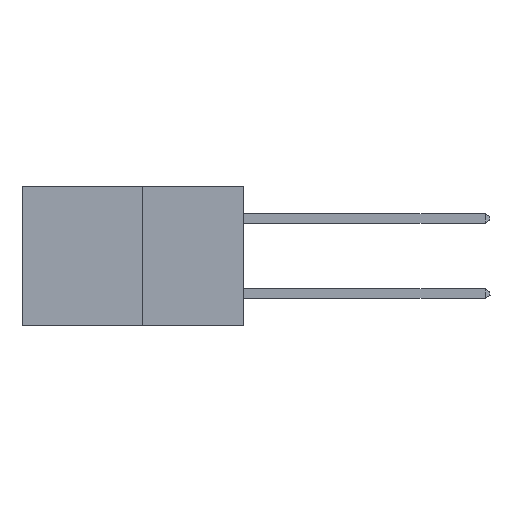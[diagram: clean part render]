
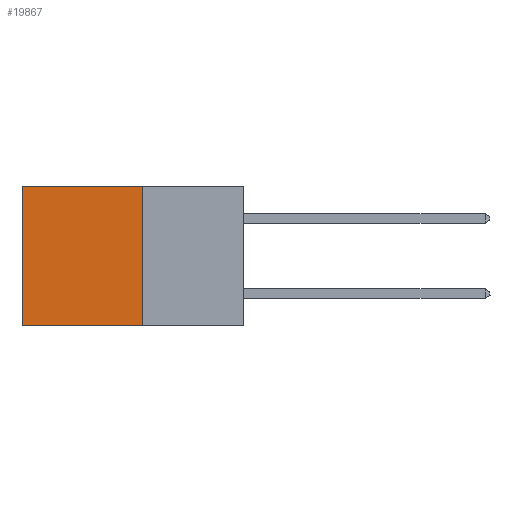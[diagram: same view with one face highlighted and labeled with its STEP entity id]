
A CAD part, left-side view. The second image highlights one B-rep face of the part: STEP entity #19867.
In plain terms, the highlighted planar face has unit normal (-1, 0, 0).
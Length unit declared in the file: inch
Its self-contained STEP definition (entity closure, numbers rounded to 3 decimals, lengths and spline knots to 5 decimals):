
#565 = DIRECTION ( 'NONE',  ( 0., 0., -1. ) ) ;
#991 = LINE ( 'NONE', #5631, #18866 ) ;
#1323 = ORIENTED_EDGE ( 'NONE', *, *, #17153, .F. ) ;
#2403 = CARTESIAN_POINT ( 'NONE',  ( 0.277, 0.27, -0.37 ) ) ;
#3775 = VERTEX_POINT ( 'NONE', #9817 ) ;
#5423 = CARTESIAN_POINT ( 'NONE',  ( 0.277, 0.59, -0.37 ) ) ;
#5631 = CARTESIAN_POINT ( 'NONE',  ( 0.277, 0.27, 0. ) ) ;
#6126 = VERTEX_POINT ( 'NONE', #5423 ) ;
#6333 = PLANE ( 'NONE',  #18625 ) ;
#7863 = LINE ( 'NONE', #8093, #21041 ) ;
#8071 = DIRECTION ( 'NONE',  ( 1., 0., 0. ) ) ;
#8093 = CARTESIAN_POINT ( 'NONE',  ( 0.277, 0.27, -0.37 ) ) ;
#9344 = VECTOR ( 'NONE', #21594, 39.37008 ) ;
#9817 = CARTESIAN_POINT ( 'NONE',  ( 0.277, 0.27, -0.37 ) ) ;
#10075 = EDGE_CURVE ( 'NONE', #13409, #3775, #15044, .T. ) ;
#10822 = DIRECTION ( 'NONE',  ( 0., 1., 0. ) ) ;
#10873 = CARTESIAN_POINT ( 'NONE',  ( 0.277, 0.59, 0. ) ) ;
#12263 = FACE_OUTER_BOUND ( 'NONE', #16210, .T. ) ;
#12900 = ORIENTED_EDGE ( 'NONE', *, *, #19788, .T. ) ;
#13336 = VERTEX_POINT ( 'NONE', #10873 ) ;
#13409 = VERTEX_POINT ( 'NONE', #21341 ) ;
#13904 = LINE ( 'NONE', #19871, #9344 ) ;
#15044 = LINE ( 'NONE', #2403, #19088 ) ;
#15312 = EDGE_CURVE ( 'NONE', #13409, #13336, #991, .T. ) ;
#16024 = ORIENTED_EDGE ( 'NONE', *, *, #10075, .F. ) ;
#16210 = EDGE_LOOP ( 'NONE', ( #12900, #1323, #16024, #19186 ) ) ;
#16567 = CARTESIAN_POINT ( 'NONE',  ( 0.277, 0.27, -0.37 ) ) ;
#17153 = EDGE_CURVE ( 'NONE', #3775, #6126, #7863, .T. ) ;
#18353 = DIRECTION ( 'NONE',  ( 0., 1., 0. ) ) ;
#18625 = AXIS2_PLACEMENT_3D ( 'NONE', #16567, #8071, #20093 ) ;
#18866 = VECTOR ( 'NONE', #10822, 39.37008 ) ;
#19088 = VECTOR ( 'NONE', #565, 39.37008 ) ;
#19186 = ORIENTED_EDGE ( 'NONE', *, *, #15312, .T. ) ;
#19788 = EDGE_CURVE ( 'NONE', #13336, #6126, #13904, .T. ) ;
#19867 = ADVANCED_FACE ( 'NONE', ( #12263 ), #6333, .F. ) ;
#19871 = CARTESIAN_POINT ( 'NONE',  ( 0.277, 0.59, -0.37 ) ) ;
#20093 = DIRECTION ( 'NONE',  ( 0., 0., -1. ) ) ;
#21041 = VECTOR ( 'NONE', #18353, 39.37008 ) ;
#21341 = CARTESIAN_POINT ( 'NONE',  ( 0.277, 0.27, 0. ) ) ;
#21594 = DIRECTION ( 'NONE',  ( 0., 0., -1. ) ) ;
